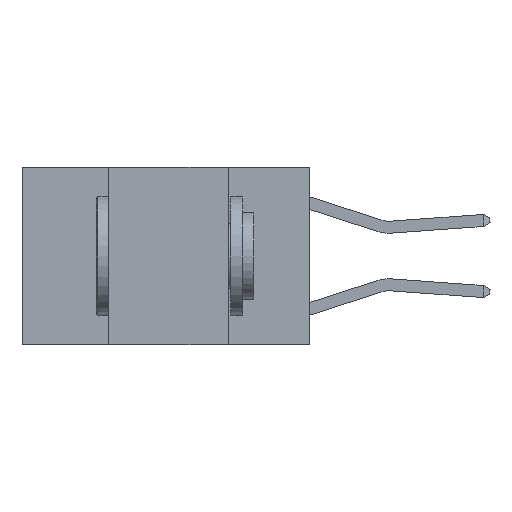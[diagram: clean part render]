
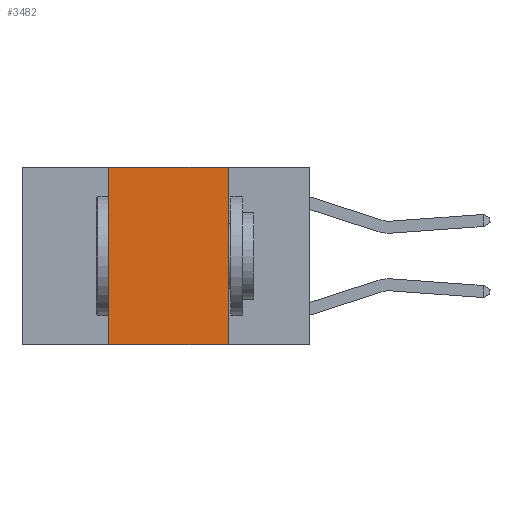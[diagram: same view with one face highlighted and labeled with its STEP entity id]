
A CAD part, left-side view. The second image highlights one B-rep face of the part: STEP entity #3482.
In plain terms, the highlighted planar face has unit normal (-1, 0, 0).
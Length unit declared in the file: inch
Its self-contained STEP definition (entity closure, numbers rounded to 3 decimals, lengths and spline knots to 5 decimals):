
#847 = FACE_OUTER_BOUND ( 'NONE', #5057, .T. ) ;
#1532 = VERTEX_POINT ( 'NONE', #6746 ) ;
#1650 = LINE ( 'NONE', #4437, #5406 ) ;
#2066 = VECTOR ( 'NONE', #8792, 39.37008 ) ;
#2087 = VECTOR ( 'NONE', #15458, 39.37008 ) ;
#2117 = CARTESIAN_POINT ( 'NONE',  ( 0., 0.6, 0. ) ) ;
#2285 = CARTESIAN_POINT ( 'NONE',  ( 0., 0.6, 0. ) ) ;
#2466 = LINE ( 'NONE', #2285, #2066 ) ;
#2601 = LINE ( 'NONE', #3783, #2087 ) ;
#2841 = VERTEX_POINT ( 'NONE', #11703 ) ;
#3482 = ADVANCED_FACE ( 'NONE', ( #847 ), #15070, .F. ) ;
#3691 = EDGE_CURVE ( 'NONE', #8944, #2841, #2466, .T. ) ;
#3783 = CARTESIAN_POINT ( 'NONE',  ( 0., 0.6, -0.37 ) ) ;
#4100 = VECTOR ( 'NONE', #9736, 39.37008 ) ;
#4378 = CARTESIAN_POINT ( 'NONE',  ( 0., 0.42, 0. ) ) ;
#4437 = CARTESIAN_POINT ( 'NONE',  ( 0., 0.17, 0. ) ) ;
#4501 = LINE ( 'NONE', #15148, #4100 ) ;
#4720 = EDGE_CURVE ( 'NONE', #1532, #7265, #2601, .T. ) ;
#5057 = EDGE_LOOP ( 'NONE', ( #12780, #13425, #11615, #9395 ) ) ;
#5406 = VECTOR ( 'NONE', #9845, 39.37008 ) ;
#6041 = DIRECTION ( 'NONE',  ( 0., 0., -1. ) ) ;
#6746 = CARTESIAN_POINT ( 'NONE',  ( 0., 0.42, -0.37 ) ) ;
#7265 = VERTEX_POINT ( 'NONE', #11008 ) ;
#8792 = DIRECTION ( 'NONE',  ( 0., -1., 0. ) ) ;
#8944 = VERTEX_POINT ( 'NONE', #4378 ) ;
#9395 = ORIENTED_EDGE ( 'NONE', *, *, #4720, .T. ) ;
#9447 = EDGE_CURVE ( 'NONE', #2841, #7265, #1650, .T. ) ;
#9736 = DIRECTION ( 'NONE',  ( 0., 0., 1. ) ) ;
#9822 = DIRECTION ( 'NONE',  ( 1., 0., 0. ) ) ;
#9845 = DIRECTION ( 'NONE',  ( 0., 0., -1. ) ) ;
#9967 = AXIS2_PLACEMENT_3D ( 'NONE', #2117, #9822, #6041 ) ;
#11008 = CARTESIAN_POINT ( 'NONE',  ( 0., 0.17, -0.37 ) ) ;
#11415 = EDGE_CURVE ( 'NONE', #1532, #8944, #4501, .T. ) ;
#11615 = ORIENTED_EDGE ( 'NONE', *, *, #11415, .F. ) ;
#11703 = CARTESIAN_POINT ( 'NONE',  ( 0., 0.17, 0. ) ) ;
#12780 = ORIENTED_EDGE ( 'NONE', *, *, #9447, .F. ) ;
#13425 = ORIENTED_EDGE ( 'NONE', *, *, #3691, .F. ) ;
#15070 = PLANE ( 'NONE',  #9967 ) ;
#15148 = CARTESIAN_POINT ( 'NONE',  ( 0., 0.42, 0. ) ) ;
#15458 = DIRECTION ( 'NONE',  ( 0., -1., 0. ) ) ;
